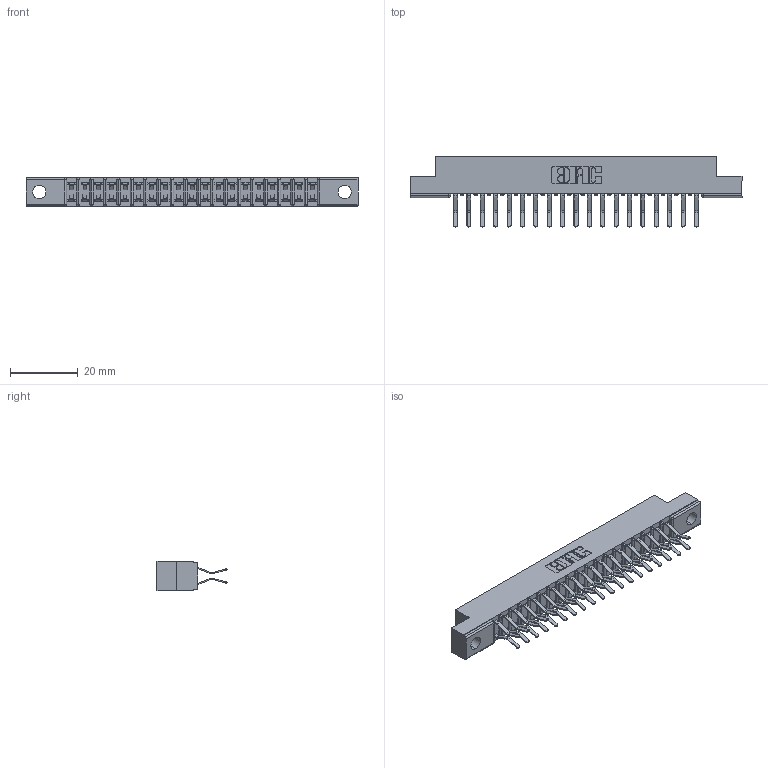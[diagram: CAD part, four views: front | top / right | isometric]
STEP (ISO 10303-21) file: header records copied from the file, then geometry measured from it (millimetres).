
FILE_DESCRIPTION (( 'STEP AP203' ), '1' );
FILE_NAME ('307-038-560-204.STEP', '2019-09-06T05:02:20', ( '' ), ( '' ), 'SwSTEP 2.0', 'SolidWorks 2016', '' );
FILE_SCHEMA (( 'CONFIG_CONTROL_DESIGN' ));
Length unit declared in the file: inch
Products named in the file (3): 307-290-001_560; 307-038-560-204; 307 Part_.156 Dia Mounting Holes
Assembly tree (39 placements, depth 2):
  307-038-560-204
    307 Part_.156 Dia Mounting Holes
    307-290-001_560  x38
Bounding box: 98.3 x 20.73 x 8.71 mm (x, y, z)
Volume: 6371.5 mm3; surface area: 11273.3 mm2
Topology: 39 solids, 39 shells, 2052 faces, 5755 edges, 3730 vertices
Faces by surface type: plane 1338, cylinder 674, sphere 40
Entity records: 20254 total; most frequent: CARTESIAN_POINT 3325, ORIENTED_EDGE 3290, DIRECTION 3259, EDGE_CURVE 1645, LINE 1259, VECTOR 1259, VERTEX_POINT 1066, AXIS2_PLACEMENT_3D 1000
